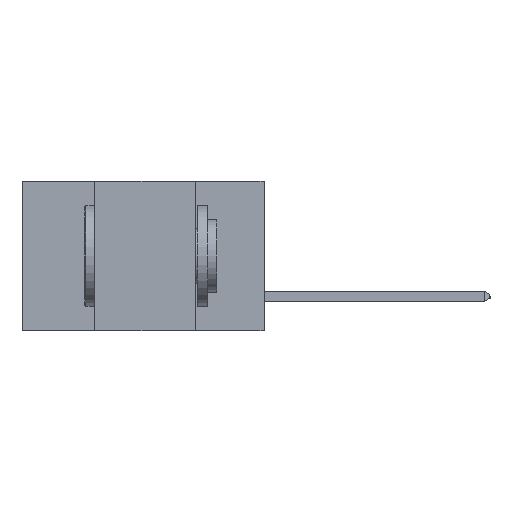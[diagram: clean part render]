
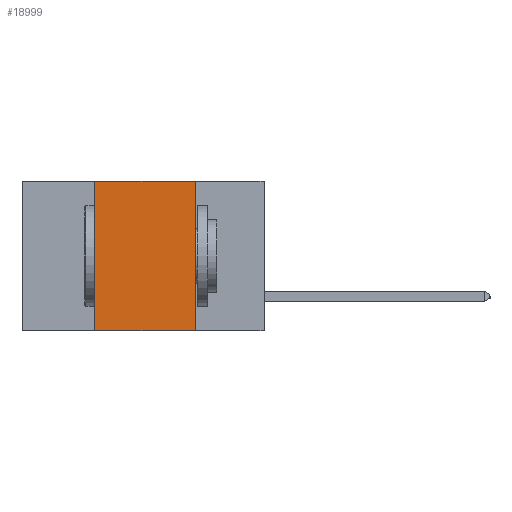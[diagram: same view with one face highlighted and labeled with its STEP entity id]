
A CAD part, left-side view. The second image highlights one B-rep face of the part: STEP entity #18999.
In plain terms, the highlighted planar face has unit normal (-1, 0, 0).
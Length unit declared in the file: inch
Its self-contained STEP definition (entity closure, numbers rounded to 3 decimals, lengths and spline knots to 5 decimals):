
#80 = CARTESIAN_POINT ( 'NONE',  ( 0., 0.42, 0. ) ) ;
#103 = DIRECTION ( 'NONE',  ( 0., 0., -1. ) ) ;
#311 = ORIENTED_EDGE ( 'NONE', *, *, #13585, .T. ) ;
#417 = EDGE_CURVE ( 'NONE', #16010, #1254, #15404, .T. ) ;
#1254 = VERTEX_POINT ( 'NONE', #8684 ) ;
#1590 = LINE ( 'NONE', #80, #13711 ) ;
#2851 = VECTOR ( 'NONE', #14621, 39.37008 ) ;
#3420 = VERTEX_POINT ( 'NONE', #19233 ) ;
#3689 = LINE ( 'NONE', #19397, #7426 ) ;
#5313 = FACE_OUTER_BOUND ( 'NONE', #19646, .T. ) ;
#5348 = VECTOR ( 'NONE', #10621, 39.37008 ) ;
#6576 = ORIENTED_EDGE ( 'NONE', *, *, #17744, .F. ) ;
#7426 = VECTOR ( 'NONE', #11782, 39.37008 ) ;
#7623 = ORIENTED_EDGE ( 'NONE', *, *, #11304, .F. ) ;
#7855 = ORIENTED_EDGE ( 'NONE', *, *, #417, .F. ) ;
#8111 = CARTESIAN_POINT ( 'NONE',  ( 0., 0.6, 0. ) ) ;
#8684 = CARTESIAN_POINT ( 'NONE',  ( 0., 0.17, -0.37 ) ) ;
#8881 = CARTESIAN_POINT ( 'NONE',  ( 0., 0.17, 0. ) ) ;
#9551 = LINE ( 'NONE', #13667, #5348 ) ;
#9624 = DIRECTION ( 'NONE',  ( 0., 0., 1. ) ) ;
#9712 = DIRECTION ( 'NONE',  ( 1., 0., 0. ) ) ;
#10621 = DIRECTION ( 'NONE',  ( 0., -1., 0. ) ) ;
#11304 = EDGE_CURVE ( 'NONE', #3420, #16010, #3689, .T. ) ;
#11782 = DIRECTION ( 'NONE',  ( 0., -1., 0. ) ) ;
#13585 = EDGE_CURVE ( 'NONE', #15200, #1254, #9551, .T. ) ;
#13667 = CARTESIAN_POINT ( 'NONE',  ( 0., 0.6, -0.37 ) ) ;
#13711 = VECTOR ( 'NONE', #9624, 39.37008 ) ;
#14621 = DIRECTION ( 'NONE',  ( 0., 0., -1. ) ) ;
#15200 = VERTEX_POINT ( 'NONE', #19277 ) ;
#15404 = LINE ( 'NONE', #19604, #2851 ) ;
#16010 = VERTEX_POINT ( 'NONE', #8881 ) ;
#16822 = AXIS2_PLACEMENT_3D ( 'NONE', #8111, #9712, #103 ) ;
#17449 = PLANE ( 'NONE',  #16822 ) ;
#17744 = EDGE_CURVE ( 'NONE', #15200, #3420, #1590, .T. ) ;
#18999 = ADVANCED_FACE ( 'NONE', ( #5313 ), #17449, .F. ) ;
#19233 = CARTESIAN_POINT ( 'NONE',  ( 0., 0.42, 0. ) ) ;
#19277 = CARTESIAN_POINT ( 'NONE',  ( 0., 0.42, -0.37 ) ) ;
#19397 = CARTESIAN_POINT ( 'NONE',  ( 0., 0.6, 0. ) ) ;
#19604 = CARTESIAN_POINT ( 'NONE',  ( 0., 0.17, 0. ) ) ;
#19646 = EDGE_LOOP ( 'NONE', ( #7855, #7623, #6576, #311 ) ) ;
